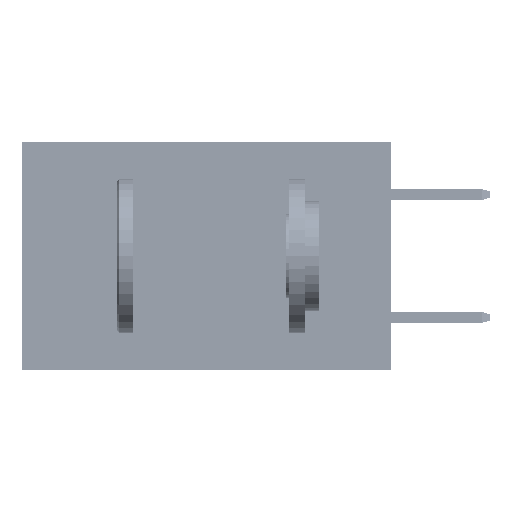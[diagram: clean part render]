
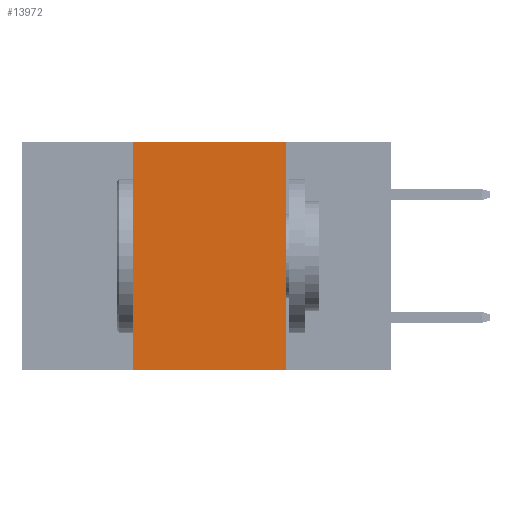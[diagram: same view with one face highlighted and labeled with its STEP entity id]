
A CAD part, left-side view. The second image highlights one B-rep face of the part: STEP entity #13972.
In plain terms, the highlighted planar face has unit normal (-1, 0, 0).
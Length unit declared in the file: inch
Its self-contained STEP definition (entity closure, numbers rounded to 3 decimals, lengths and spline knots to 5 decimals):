
#485 = VERTEX_POINT ( 'NONE', #16722 ) ;
#2735 = DIRECTION ( 'NONE',  ( 0., 0., -1. ) ) ;
#3625 = DIRECTION ( 'NONE',  ( 0., 0., 1. ) ) ;
#3819 = EDGE_CURVE ( 'NONE', #13193, #485, #28539, .T. ) ;
#4072 = CARTESIAN_POINT ( 'NONE',  ( 0., 0.6, 0. ) ) ;
#4095 = VECTOR ( 'NONE', #3625, 39.37008 ) ;
#5768 = LINE ( 'NONE', #20449, #19027 ) ;
#7010 = ORIENTED_EDGE ( 'NONE', *, *, #43969, .T. ) ;
#9902 = EDGE_CURVE ( 'NONE', #20563, #29746, #18469, .T. ) ;
#10743 = PLANE ( 'NONE',  #44033 ) ;
#11471 = DIRECTION ( 'NONE',  ( 0., -1., 0. ) ) ;
#13193 = VERTEX_POINT ( 'NONE', #27487 ) ;
#13972 = ADVANCED_FACE ( 'NONE', ( #34238 ), #10743, .F. ) ;
#15092 = ORIENTED_EDGE ( 'NONE', *, *, #3819, .F. ) ;
#16722 = CARTESIAN_POINT ( 'NONE',  ( 0., 0.17, -0.37 ) ) ;
#17628 = CARTESIAN_POINT ( 'NONE',  ( 0., 0.42, 0. ) ) ;
#18469 = LINE ( 'NONE', #36556, #4095 ) ;
#18812 = VECTOR ( 'NONE', #2735, 39.37008 ) ;
#19027 = VECTOR ( 'NONE', #27807, 39.37008 ) ;
#19123 = EDGE_CURVE ( 'NONE', #29746, #13193, #25155, .T. ) ;
#20449 = CARTESIAN_POINT ( 'NONE',  ( 0., 0.6, -0.37 ) ) ;
#20563 = VERTEX_POINT ( 'NONE', #23675 ) ;
#20995 = ORIENTED_EDGE ( 'NONE', *, *, #19123, .F. ) ;
#21797 = DIRECTION ( 'NONE',  ( 1., 0., 0. ) ) ;
#21955 = DIRECTION ( 'NONE',  ( 0., 0., -1. ) ) ;
#23675 = CARTESIAN_POINT ( 'NONE',  ( 0., 0.42, -0.37 ) ) ;
#25155 = LINE ( 'NONE', #4072, #28000 ) ;
#27487 = CARTESIAN_POINT ( 'NONE',  ( 0., 0.17, 0. ) ) ;
#27807 = DIRECTION ( 'NONE',  ( 0., -1., 0. ) ) ;
#28000 = VECTOR ( 'NONE', #11471, 39.37008 ) ;
#28004 = ORIENTED_EDGE ( 'NONE', *, *, #9902, .F. ) ;
#28539 = LINE ( 'NONE', #39184, #18812 ) ;
#29746 = VERTEX_POINT ( 'NONE', #17628 ) ;
#34238 = FACE_OUTER_BOUND ( 'NONE', #42942, .T. ) ;
#36556 = CARTESIAN_POINT ( 'NONE',  ( 0., 0.42, 0. ) ) ;
#36743 = CARTESIAN_POINT ( 'NONE',  ( 0., 0.6, 0. ) ) ;
#39184 = CARTESIAN_POINT ( 'NONE',  ( 0., 0.17, 0. ) ) ;
#42942 = EDGE_LOOP ( 'NONE', ( #15092, #20995, #28004, #7010 ) ) ;
#43969 = EDGE_CURVE ( 'NONE', #20563, #485, #5768, .T. ) ;
#44033 = AXIS2_PLACEMENT_3D ( 'NONE', #36743, #21797, #21955 ) ;
